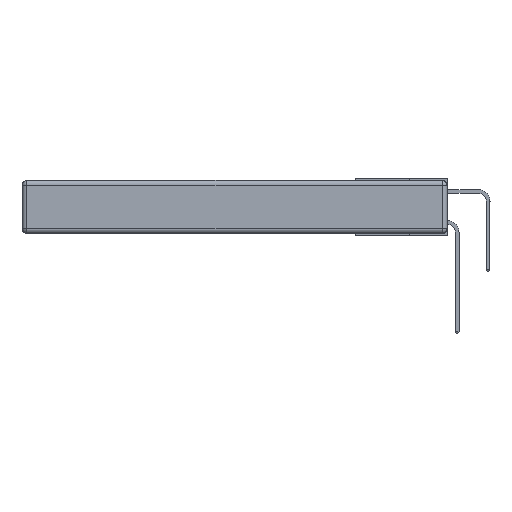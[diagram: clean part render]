
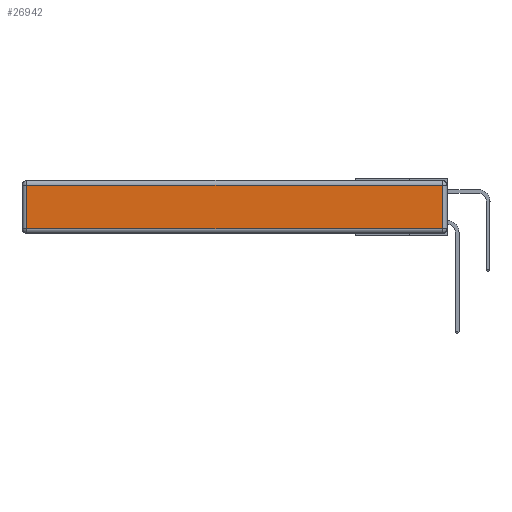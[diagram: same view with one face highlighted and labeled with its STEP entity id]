
A CAD part, left-side view. The second image highlights one B-rep face of the part: STEP entity #26942.
In plain terms, the highlighted planar face has unit normal (-1, 0, 0).
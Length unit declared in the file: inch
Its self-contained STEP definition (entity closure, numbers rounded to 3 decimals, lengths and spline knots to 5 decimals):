
#520 = DIRECTION ( 'NONE',  ( 0., 0., -1. ) ) ;
#2075 = DIRECTION ( 'NONE',  ( 0., 0., 1. ) ) ;
#2144 = VERTEX_POINT ( 'NONE', #15648 ) ;
#2531 = VERTEX_POINT ( 'NONE', #19225 ) ;
#2632 = EDGE_CURVE ( 'NONE', #15936, #2531, #5464, .T. ) ;
#3086 = AXIS2_PLACEMENT_3D ( 'NONE', #24707, #29358, #2075 ) ;
#3100 = CARTESIAN_POINT ( 'NONE',  ( 0., 0.03, -0.343 ) ) ;
#3960 = EDGE_CURVE ( 'NONE', #2144, #15936, #15798, .T. ) ;
#4518 = CARTESIAN_POINT ( 'NONE',  ( 0., 0., -0.313 ) ) ;
#5464 = LINE ( 'NONE', #10934, #9773 ) ;
#6682 = ORIENTED_EDGE ( 'NONE', *, *, #19217, .T. ) ;
#7470 = FACE_OUTER_BOUND ( 'NONE', #22868, .T. ) ;
#7556 = DIRECTION ( 'NONE',  ( 0., 0., 1. ) ) ;
#9145 = LINE ( 'NONE', #14164, #21195 ) ;
#9773 = VECTOR ( 'NONE', #22009, 39.37008 ) ;
#10095 = VECTOR ( 'NONE', #7556, 39.37008 ) ;
#10934 = CARTESIAN_POINT ( 'NONE',  ( 0., 2.75, -0.03 ) ) ;
#13414 = PLANE ( 'NONE',  #3086 ) ;
#14164 = CARTESIAN_POINT ( 'NONE',  ( 0., 2.72, -0.343 ) ) ;
#14866 = ORIENTED_EDGE ( 'NONE', *, *, #28456, .T. ) ;
#15648 = CARTESIAN_POINT ( 'NONE',  ( 0., 0.03, -0.313 ) ) ;
#15798 = LINE ( 'NONE', #3100, #10095 ) ;
#15936 = VERTEX_POINT ( 'NONE', #26025 ) ;
#18273 = CARTESIAN_POINT ( 'NONE',  ( 0., 2.72, -0.313 ) ) ;
#19217 = EDGE_CURVE ( 'NONE', #2531, #21034, #9145, .T. ) ;
#19225 = CARTESIAN_POINT ( 'NONE',  ( 0., 2.72, -0.03 ) ) ;
#19419 = LINE ( 'NONE', #4518, #23022 ) ;
#20455 = ORIENTED_EDGE ( 'NONE', *, *, #2632, .T. ) ;
#21034 = VERTEX_POINT ( 'NONE', #18273 ) ;
#21195 = VECTOR ( 'NONE', #520, 39.37008 ) ;
#21709 = ORIENTED_EDGE ( 'NONE', *, *, #3960, .T. ) ;
#22009 = DIRECTION ( 'NONE',  ( 0., 1., 0. ) ) ;
#22599 = DIRECTION ( 'NONE',  ( 0., -1., 0. ) ) ;
#22868 = EDGE_LOOP ( 'NONE', ( #14866, #21709, #20455, #6682 ) ) ;
#23022 = VECTOR ( 'NONE', #22599, 39.37008 ) ;
#24707 = CARTESIAN_POINT ( 'NONE',  ( 0., 0., -0.343 ) ) ;
#26025 = CARTESIAN_POINT ( 'NONE',  ( 0., 0.03, -0.03 ) ) ;
#26942 = ADVANCED_FACE ( 'NONE', ( #7470 ), #13414, .T. ) ;
#28456 = EDGE_CURVE ( 'NONE', #21034, #2144, #19419, .T. ) ;
#29358 = DIRECTION ( 'NONE',  ( -1., 0., 0. ) ) ;
